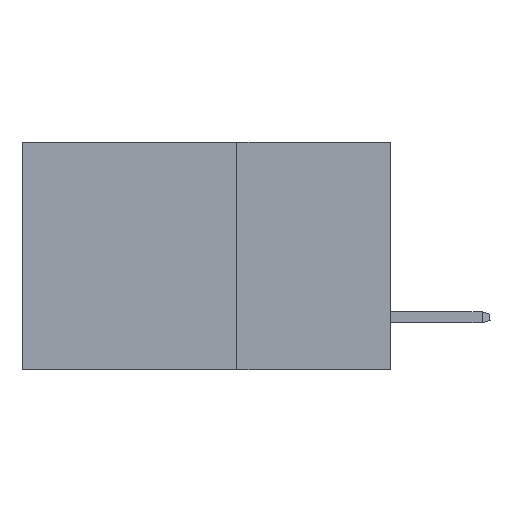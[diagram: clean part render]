
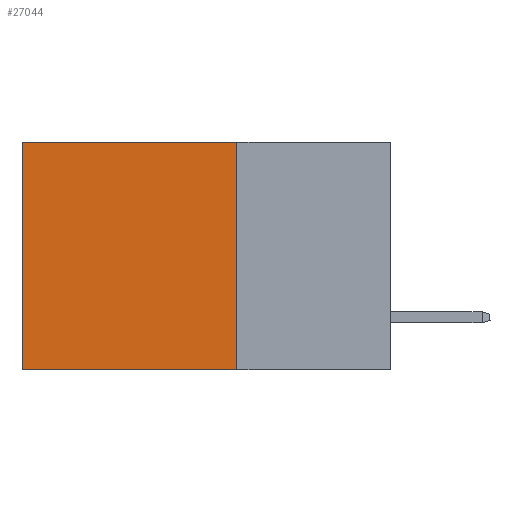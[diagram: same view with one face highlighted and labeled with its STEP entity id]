
A CAD part, left-side view. The second image highlights one B-rep face of the part: STEP entity #27044.
In plain terms, the highlighted planar face has unit normal (-1, 0, 0).
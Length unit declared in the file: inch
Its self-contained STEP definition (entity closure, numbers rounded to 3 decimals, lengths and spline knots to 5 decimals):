
#849 = DIRECTION ( 'NONE',  ( 0., 0., -1. ) ) ;
#1044 = LINE ( 'NONE', #30703, #5399 ) ;
#1689 = VERTEX_POINT ( 'NONE', #12582 ) ;
#2123 = CARTESIAN_POINT ( 'NONE',  ( 0.2875, 0.25, -0.37 ) ) ;
#2559 = CARTESIAN_POINT ( 'NONE',  ( 0.2875, 0.25, -0.37 ) ) ;
#2713 = VERTEX_POINT ( 'NONE', #17240 ) ;
#5399 = VECTOR ( 'NONE', #15447, 39.37008 ) ;
#5655 = CARTESIAN_POINT ( 'NONE',  ( 0.2875, 0.6, -0.37 ) ) ;
#9010 = VECTOR ( 'NONE', #12876, 39.37008 ) ;
#10789 = PLANE ( 'NONE',  #17718 ) ;
#10796 = CARTESIAN_POINT ( 'NONE',  ( 0.2875, 0.25, 0. ) ) ;
#12530 = EDGE_CURVE ( 'NONE', #17102, #17256, #15877, .T. ) ;
#12582 = CARTESIAN_POINT ( 'NONE',  ( 0.2875, 0.6, 0. ) ) ;
#12768 = CARTESIAN_POINT ( 'NONE',  ( 0.2875, 0.6, 0. ) ) ;
#12876 = DIRECTION ( 'NONE',  ( 0., 0., -1. ) ) ;
#14278 = VECTOR ( 'NONE', #24554, 39.37008 ) ;
#14987 = VECTOR ( 'NONE', #849, 39.37008 ) ;
#15447 = DIRECTION ( 'NONE',  ( 0., 1., 0. ) ) ;
#15877 = LINE ( 'NONE', #2123, #14278 ) ;
#16105 = DIRECTION ( 'NONE',  ( 0., 0., -1. ) ) ;
#16558 = LINE ( 'NONE', #12768, #9010 ) ;
#16926 = ORIENTED_EDGE ( 'NONE', *, *, #30854, .T. ) ;
#16955 = LINE ( 'NONE', #10796, #14987 ) ;
#17046 = EDGE_LOOP ( 'NONE', ( #16926, #24910, #30229, #27905 ) ) ;
#17102 = VERTEX_POINT ( 'NONE', #2559 ) ;
#17240 = CARTESIAN_POINT ( 'NONE',  ( 0.2875, 0.25, 0. ) ) ;
#17256 = VERTEX_POINT ( 'NONE', #5655 ) ;
#17718 = AXIS2_PLACEMENT_3D ( 'NONE', #18455, #31240, #16105 ) ;
#18455 = CARTESIAN_POINT ( 'NONE',  ( 0.2875, 0.25, 0. ) ) ;
#20482 = EDGE_CURVE ( 'NONE', #2713, #17102, #16955, .T. ) ;
#21259 = EDGE_CURVE ( 'NONE', #2713, #1689, #1044, .T. ) ;
#24554 = DIRECTION ( 'NONE',  ( 0., 1., 0. ) ) ;
#24910 = ORIENTED_EDGE ( 'NONE', *, *, #12530, .F. ) ;
#27044 = ADVANCED_FACE ( 'NONE', ( #30076 ), #10789, .F. ) ;
#27905 = ORIENTED_EDGE ( 'NONE', *, *, #21259, .T. ) ;
#30076 = FACE_OUTER_BOUND ( 'NONE', #17046, .T. ) ;
#30229 = ORIENTED_EDGE ( 'NONE', *, *, #20482, .F. ) ;
#30703 = CARTESIAN_POINT ( 'NONE',  ( 0.2875, 0.25, 0. ) ) ;
#30854 = EDGE_CURVE ( 'NONE', #1689, #17256, #16558, .T. ) ;
#31240 = DIRECTION ( 'NONE',  ( 1., 0., 0. ) ) ;
